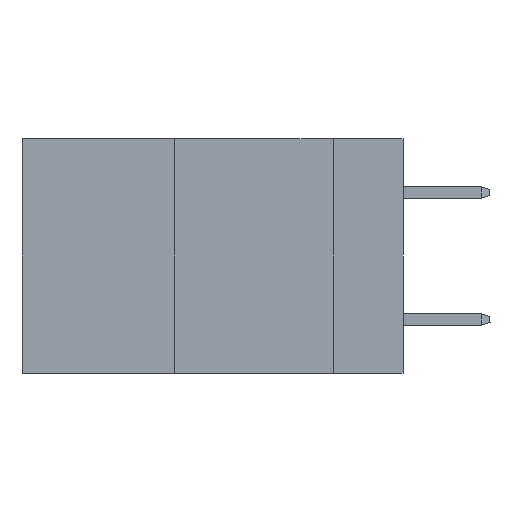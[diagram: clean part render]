
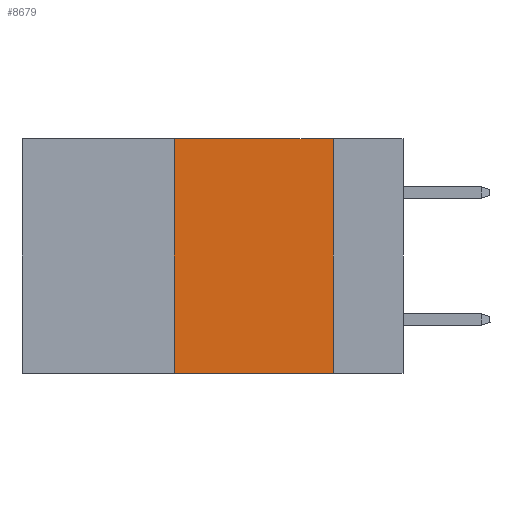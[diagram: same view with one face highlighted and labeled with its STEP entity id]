
A CAD part, left-side view. The second image highlights one B-rep face of the part: STEP entity #8679.
In plain terms, the highlighted planar face has unit normal (-1, 0, 0).
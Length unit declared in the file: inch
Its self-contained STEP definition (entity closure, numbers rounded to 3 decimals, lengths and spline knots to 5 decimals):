
#34 = EDGE_CURVE ( 'NONE', #7593, #12430, #453, .T. ) ;
#453 = LINE ( 'NONE', #5899, #3227 ) ;
#1043 = PLANE ( 'NONE',  #4262 ) ;
#2153 = VERTEX_POINT ( 'NONE', #5686 ) ;
#2322 = CARTESIAN_POINT ( 'NONE',  ( 0., 0.36, 0. ) ) ;
#2665 = VECTOR ( 'NONE', #10627, 39.37008 ) ;
#2861 = ORIENTED_EDGE ( 'NONE', *, *, #16465, .F. ) ;
#3114 = EDGE_CURVE ( 'NONE', #2153, #12430, #11401, .T. ) ;
#3218 = DIRECTION ( 'NONE',  ( 0., -1., 0. ) ) ;
#3227 = VECTOR ( 'NONE', #3218, 39.37008 ) ;
#3463 = CARTESIAN_POINT ( 'NONE',  ( 0., 0.11, 0. ) ) ;
#3740 = VECTOR ( 'NONE', #16796, 39.37008 ) ;
#4017 = CARTESIAN_POINT ( 'NONE',  ( 0., 0.6, 0. ) ) ;
#4262 = AXIS2_PLACEMENT_3D ( 'NONE', #14696, #12999, #17343 ) ;
#4410 = VECTOR ( 'NONE', #7415, 39.37008 ) ;
#4688 = CARTESIAN_POINT ( 'NONE',  ( 0., 0.36, 0. ) ) ;
#5686 = CARTESIAN_POINT ( 'NONE',  ( 0., 0.11, 0. ) ) ;
#5899 = CARTESIAN_POINT ( 'NONE',  ( 0., 0.6, -0.37 ) ) ;
#7415 = DIRECTION ( 'NONE',  ( 0., 0., 1. ) ) ;
#7568 = FACE_OUTER_BOUND ( 'NONE', #15685, .T. ) ;
#7589 = LINE ( 'NONE', #2322, #4410 ) ;
#7593 = VERTEX_POINT ( 'NONE', #16529 ) ;
#8679 = ADVANCED_FACE ( 'NONE', ( #7568 ), #1043, .F. ) ;
#10214 = ORIENTED_EDGE ( 'NONE', *, *, #34, .T. ) ;
#10627 = DIRECTION ( 'NONE',  ( 0., -1., 0. ) ) ;
#11047 = ORIENTED_EDGE ( 'NONE', *, *, #3114, .F. ) ;
#11401 = LINE ( 'NONE', #3463, #3740 ) ;
#12187 = VERTEX_POINT ( 'NONE', #4688 ) ;
#12430 = VERTEX_POINT ( 'NONE', #14222 ) ;
#12999 = DIRECTION ( 'NONE',  ( 1., 0., 0. ) ) ;
#13289 = ORIENTED_EDGE ( 'NONE', *, *, #14590, .F. ) ;
#14222 = CARTESIAN_POINT ( 'NONE',  ( 0., 0.11, -0.37 ) ) ;
#14590 = EDGE_CURVE ( 'NONE', #12187, #2153, #17359, .T. ) ;
#14696 = CARTESIAN_POINT ( 'NONE',  ( 0., 0.6, 0. ) ) ;
#15685 = EDGE_LOOP ( 'NONE', ( #11047, #13289, #2861, #10214 ) ) ;
#16465 = EDGE_CURVE ( 'NONE', #7593, #12187, #7589, .T. ) ;
#16529 = CARTESIAN_POINT ( 'NONE',  ( 0., 0.36, -0.37 ) ) ;
#16796 = DIRECTION ( 'NONE',  ( 0., 0., -1. ) ) ;
#17343 = DIRECTION ( 'NONE',  ( 0., 0., -1. ) ) ;
#17359 = LINE ( 'NONE', #4017, #2665 ) ;
